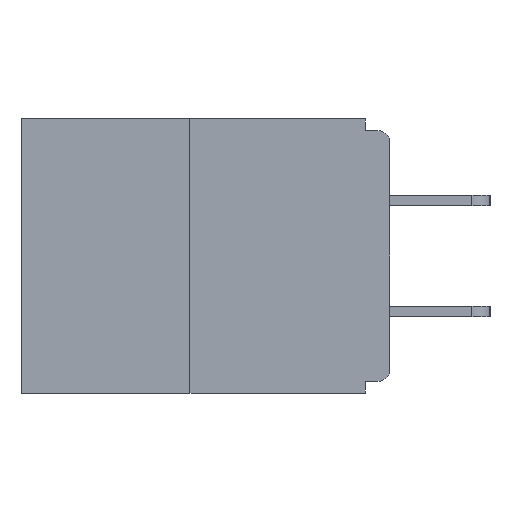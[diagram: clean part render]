
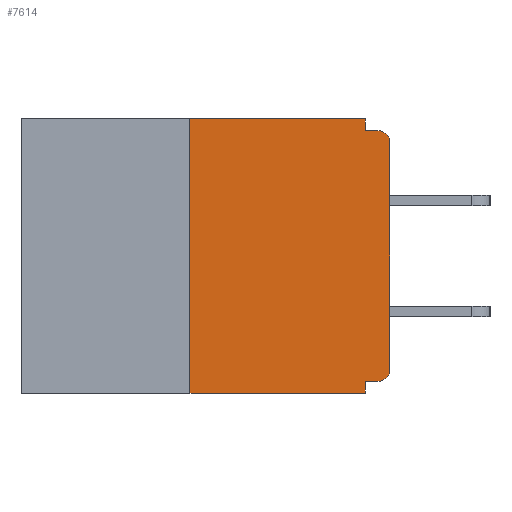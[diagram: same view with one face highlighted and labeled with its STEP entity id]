
A CAD part, left-side view. The second image highlights one B-rep face of the part: STEP entity #7614.
In plain terms, the highlighted planar face has unit normal (-1, 0, 0).
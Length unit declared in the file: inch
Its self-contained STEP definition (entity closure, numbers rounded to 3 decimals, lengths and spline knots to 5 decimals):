
#474 = EDGE_CURVE ( 'NONE', #12247, #2113, #14044, .T. ) ;
#614 = ORIENTED_EDGE ( 'NONE', *, *, #14200, .T. ) ;
#632 = VECTOR ( 'NONE', #935, 39.37008 ) ;
#888 = CARTESIAN_POINT ( 'NONE',  ( 0., 0.031, 0. ) ) ;
#935 = DIRECTION ( 'NONE',  ( 0., 0., -1. ) ) ;
#1835 = DIRECTION ( 'NONE',  ( 0., 0., -1. ) ) ;
#2113 = VERTEX_POINT ( 'NONE', #10645 ) ;
#2896 = AXIS2_PLACEMENT_3D ( 'NONE', #8116, #8269, #1835 ) ;
#3154 = AXIS2_PLACEMENT_3D ( 'NONE', #8931, #14150, #7636 ) ;
#3213 = EDGE_LOOP ( 'NONE', ( #6928, #10371, #614, #14018, #7179, #11437, #10318, #9348, #8768, #5440 ) ) ;
#4705 = VECTOR ( 'NONE', #8201, 39.37008 ) ;
#4814 = CARTESIAN_POINT ( 'NONE',  ( 0., 0., -0.03 ) ) ;
#4994 = AXIS2_PLACEMENT_3D ( 'NONE', #5187, #13013, #11724 ) ;
#5136 = VERTEX_POINT ( 'NONE', #9025 ) ;
#5187 = CARTESIAN_POINT ( 'NONE',  ( 0., 0.46, 0. ) ) ;
#5300 = EDGE_CURVE ( 'NONE', #5582, #13482, #13316, .T. ) ;
#5334 = DIRECTION ( 'NONE',  ( 0., 1., 0. ) ) ;
#5440 = ORIENTED_EDGE ( 'NONE', *, *, #474, .F. ) ;
#5582 = VERTEX_POINT ( 'NONE', #12709 ) ;
#5617 = VECTOR ( 'NONE', #16799, 39.37008 ) ;
#5685 = EDGE_CURVE ( 'NONE', #6614, #16678, #14383, .T. ) ;
#5829 = VECTOR ( 'NONE', #11496, 39.37008 ) ;
#6264 = CARTESIAN_POINT ( 'NONE',  ( 0., 0.031, -0.328 ) ) ;
#6268 = LINE ( 'NONE', #9085, #5829 ) ;
#6375 = CARTESIAN_POINT ( 'NONE',  ( 0., 0.015, -0.015 ) ) ;
#6578 = EDGE_CURVE ( 'NONE', #2113, #16678, #8767, .T. ) ;
#6587 = VERTEX_POINT ( 'NONE', #8501 ) ;
#6614 = VERTEX_POINT ( 'NONE', #4814 ) ;
#6928 = ORIENTED_EDGE ( 'NONE', *, *, #14201, .F. ) ;
#6953 = VECTOR ( 'NONE', #15249, 39.37008 ) ;
#7179 = ORIENTED_EDGE ( 'NONE', *, *, #5300, .F. ) ;
#7281 = LINE ( 'NONE', #8737, #6953 ) ;
#7292 = CIRCLE ( 'NONE', #2896, 0.015 ) ;
#7614 = ADVANCED_FACE ( 'NONE', ( #14267 ), #16954, .F. ) ;
#7636 = DIRECTION ( 'NONE',  ( 0., 0., -1. ) ) ;
#7816 = CARTESIAN_POINT ( 'NONE',  ( 0., 0.25, 0. ) ) ;
#8116 = CARTESIAN_POINT ( 'NONE',  ( 0., 0.015, -0.313 ) ) ;
#8128 = CARTESIAN_POINT ( 'NONE',  ( 0., 0.46, -0.343 ) ) ;
#8201 = DIRECTION ( 'NONE',  ( 0., -1., 0. ) ) ;
#8269 = DIRECTION ( 'NONE',  ( -1., 0., 0. ) ) ;
#8501 = CARTESIAN_POINT ( 'NONE',  ( 0., 0., -0.313 ) ) ;
#8593 = CARTESIAN_POINT ( 'NONE',  ( 0., 0., -0.015 ) ) ;
#8737 = CARTESIAN_POINT ( 'NONE',  ( 0., 0., 0. ) ) ;
#8767 = LINE ( 'NONE', #8593, #11972 ) ;
#8768 = ORIENTED_EDGE ( 'NONE', *, *, #6578, .F. ) ;
#8931 = CARTESIAN_POINT ( 'NONE',  ( 0., 0.015, -0.03 ) ) ;
#9025 = CARTESIAN_POINT ( 'NONE',  ( 0., 0.25, -0.343 ) ) ;
#9085 = CARTESIAN_POINT ( 'NONE',  ( 0., 0.25, 0. ) ) ;
#9340 = EDGE_CURVE ( 'NONE', #5136, #15522, #6268, .T. ) ;
#9348 = ORIENTED_EDGE ( 'NONE', *, *, #5685, .T. ) ;
#9396 = VECTOR ( 'NONE', #5334, 39.37008 ) ;
#9404 = LINE ( 'NONE', #8128, #11559 ) ;
#9491 = DIRECTION ( 'NONE',  ( 0., -1., 0. ) ) ;
#10138 = DIRECTION ( 'NONE',  ( 0., -1., 0. ) ) ;
#10318 = ORIENTED_EDGE ( 'NONE', *, *, #16208, .T. ) ;
#10371 = ORIENTED_EDGE ( 'NONE', *, *, #9340, .F. ) ;
#10645 = CARTESIAN_POINT ( 'NONE',  ( 0., 0.031, -0.015 ) ) ;
#10863 = CARTESIAN_POINT ( 'NONE',  ( 0., 0.46, 0. ) ) ;
#11396 = EDGE_CURVE ( 'NONE', #13482, #16313, #11656, .T. ) ;
#11437 = ORIENTED_EDGE ( 'NONE', *, *, #12058, .T. ) ;
#11496 = DIRECTION ( 'NONE',  ( 0., 0., 1. ) ) ;
#11556 = CARTESIAN_POINT ( 'NONE',  ( 0., 0.031, -0.343 ) ) ;
#11559 = VECTOR ( 'NONE', #9491, 39.37008 ) ;
#11656 = LINE ( 'NONE', #11556, #5617 ) ;
#11724 = DIRECTION ( 'NONE',  ( 0., 0., -1. ) ) ;
#11972 = VECTOR ( 'NONE', #10138, 39.37008 ) ;
#12058 = EDGE_CURVE ( 'NONE', #5582, #6587, #7292, .T. ) ;
#12247 = VERTEX_POINT ( 'NONE', #888 ) ;
#12709 = CARTESIAN_POINT ( 'NONE',  ( 0., 0.015, -0.328 ) ) ;
#13013 = DIRECTION ( 'NONE',  ( 1., 0., 0. ) ) ;
#13316 = LINE ( 'NONE', #15981, #9396 ) ;
#13482 = VERTEX_POINT ( 'NONE', #6264 ) ;
#13794 = CARTESIAN_POINT ( 'NONE',  ( 0., 0.031, 0. ) ) ;
#14018 = ORIENTED_EDGE ( 'NONE', *, *, #11396, .F. ) ;
#14033 = CARTESIAN_POINT ( 'NONE',  ( 0., 0.031, -0.343 ) ) ;
#14044 = LINE ( 'NONE', #13794, #632 ) ;
#14150 = DIRECTION ( 'NONE',  ( -1., 0., 0. ) ) ;
#14200 = EDGE_CURVE ( 'NONE', #5136, #16313, #9404, .T. ) ;
#14201 = EDGE_CURVE ( 'NONE', #15522, #12247, #14707, .T. ) ;
#14267 = FACE_OUTER_BOUND ( 'NONE', #3213, .T. ) ;
#14383 = CIRCLE ( 'NONE', #3154, 0.015 ) ;
#14707 = LINE ( 'NONE', #10863, #4705 ) ;
#15249 = DIRECTION ( 'NONE',  ( 0., 0., 1. ) ) ;
#15522 = VERTEX_POINT ( 'NONE', #7816 ) ;
#15981 = CARTESIAN_POINT ( 'NONE',  ( 0., 0., -0.328 ) ) ;
#16208 = EDGE_CURVE ( 'NONE', #6587, #6614, #7281, .T. ) ;
#16313 = VERTEX_POINT ( 'NONE', #14033 ) ;
#16678 = VERTEX_POINT ( 'NONE', #6375 ) ;
#16799 = DIRECTION ( 'NONE',  ( 0., 0., -1. ) ) ;
#16954 = PLANE ( 'NONE',  #4994 ) ;
